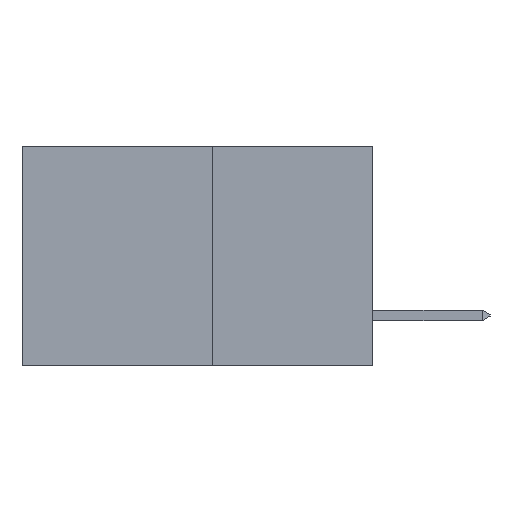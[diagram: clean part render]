
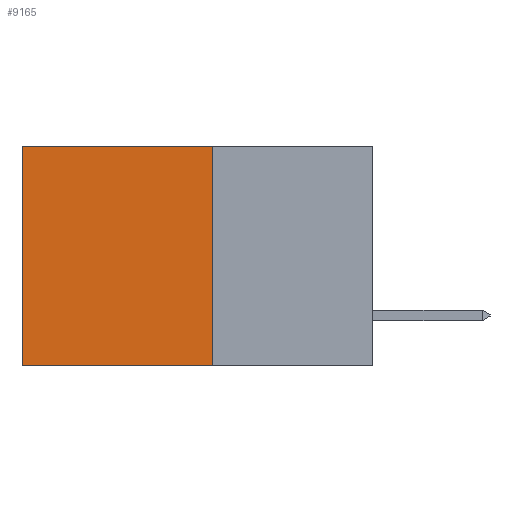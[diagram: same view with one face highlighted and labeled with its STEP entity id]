
A CAD part, left-side view. The second image highlights one B-rep face of the part: STEP entity #9165.
In plain terms, the highlighted planar face has unit normal (-1, 0, 0).
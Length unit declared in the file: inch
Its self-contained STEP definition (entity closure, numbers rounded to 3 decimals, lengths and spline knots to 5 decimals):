
#140 = VERTEX_POINT ( 'NONE', #24696 ) ;
#947 = AXIS2_PLACEMENT_3D ( 'NONE', #5368, #11642, #25868 ) ;
#2246 = ORIENTED_EDGE ( 'NONE', *, *, #4489, .T. ) ;
#2380 = LINE ( 'NONE', #7507, #12798 ) ;
#3088 = CARTESIAN_POINT ( 'NONE',  ( 0.277, 0.59, -0.37 ) ) ;
#3608 = ORIENTED_EDGE ( 'NONE', *, *, #14931, .F. ) ;
#4489 = EDGE_CURVE ( 'NONE', #17114, #140, #8885, .T. ) ;
#5368 = CARTESIAN_POINT ( 'NONE',  ( 0.277, 0.27, -0.37 ) ) ;
#7507 = CARTESIAN_POINT ( 'NONE',  ( 0.277, 0.27, -0.37 ) ) ;
#8014 = FACE_OUTER_BOUND ( 'NONE', #19772, .T. ) ;
#8885 = LINE ( 'NONE', #17211, #17239 ) ;
#9165 = ADVANCED_FACE ( 'NONE', ( #8014 ), #23863, .F. ) ;
#9599 = DIRECTION ( 'NONE',  ( 0., 1., 0. ) ) ;
#10414 = EDGE_CURVE ( 'NONE', #12250, #24838, #2380, .T. ) ;
#11541 = ORIENTED_EDGE ( 'NONE', *, *, #10414, .F. ) ;
#11634 = DIRECTION ( 'NONE',  ( 0., 0., -1. ) ) ;
#11642 = DIRECTION ( 'NONE',  ( 1., 0., 0. ) ) ;
#12250 = VERTEX_POINT ( 'NONE', #26088 ) ;
#12798 = VECTOR ( 'NONE', #9599, 39.37008 ) ;
#13904 = ORIENTED_EDGE ( 'NONE', *, *, #14860, .T. ) ;
#14860 = EDGE_CURVE ( 'NONE', #140, #24838, #22090, .T. ) ;
#14931 = EDGE_CURVE ( 'NONE', #17114, #12250, #19555, .T. ) ;
#15385 = VECTOR ( 'NONE', #19611, 39.37008 ) ;
#17114 = VERTEX_POINT ( 'NONE', #22337 ) ;
#17174 = DIRECTION ( 'NONE',  ( 0., 1., 0. ) ) ;
#17211 = CARTESIAN_POINT ( 'NONE',  ( 0.277, 0.27, 0. ) ) ;
#17239 = VECTOR ( 'NONE', #17174, 39.37008 ) ;
#18912 = VECTOR ( 'NONE', #11634, 39.37008 ) ;
#19555 = LINE ( 'NONE', #25856, #18912 ) ;
#19611 = DIRECTION ( 'NONE',  ( 0., 0., -1. ) ) ;
#19772 = EDGE_LOOP ( 'NONE', ( #13904, #11541, #3608, #2246 ) ) ;
#22090 = LINE ( 'NONE', #3088, #15385 ) ;
#22337 = CARTESIAN_POINT ( 'NONE',  ( 0.277, 0.27, 0. ) ) ;
#22973 = CARTESIAN_POINT ( 'NONE',  ( 0.277, 0.59, -0.37 ) ) ;
#23863 = PLANE ( 'NONE',  #947 ) ;
#24696 = CARTESIAN_POINT ( 'NONE',  ( 0.277, 0.59, 0. ) ) ;
#24838 = VERTEX_POINT ( 'NONE', #22973 ) ;
#25856 = CARTESIAN_POINT ( 'NONE',  ( 0.277, 0.27, -0.37 ) ) ;
#25868 = DIRECTION ( 'NONE',  ( 0., 0., -1. ) ) ;
#26088 = CARTESIAN_POINT ( 'NONE',  ( 0.277, 0.27, -0.37 ) ) ;
